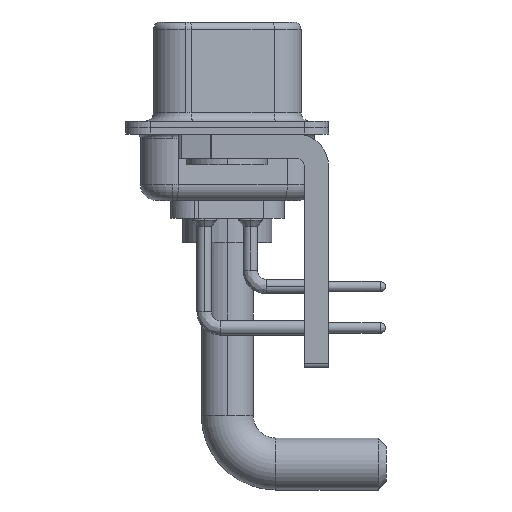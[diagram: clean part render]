
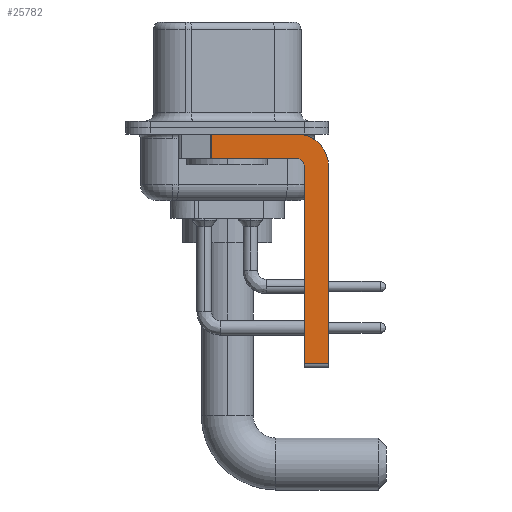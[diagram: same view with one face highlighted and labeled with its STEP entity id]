
A CAD part, left-side view. The second image highlights one B-rep face of the part: STEP entity #25782.
In plain terms, the highlighted planar face has unit normal (-1, 0, 0).
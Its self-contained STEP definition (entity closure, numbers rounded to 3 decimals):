
#176 = DIRECTION ( 'NONE',  ( -1., 0., 0. ) ) ;
#383 = EDGE_CURVE ( 'NONE', #3870, #25804, #3470, .T. ) ;
#415 = CARTESIAN_POINT ( 'NONE',  ( -2.9, -4.75, -2.4 ) ) ;
#461 = DIRECTION ( 'NONE',  ( 0., 0., 1. ) ) ;
#722 = ORIENTED_EDGE ( 'NONE', *, *, #26413, .F. ) ;
#1098 = AXIS2_PLACEMENT_3D ( 'NONE', #14844, #8532, #25747 ) ;
#1324 = CARTESIAN_POINT ( 'NONE',  ( -2.9, -4.75, -14.55 ) ) ;
#1510 = DIRECTION ( 'NONE',  ( 0., 1., 0. ) ) ;
#1531 = VERTEX_POINT ( 'NONE', #12823 ) ;
#1748 = DIRECTION ( 'NONE',  ( 1., 0., 0. ) ) ;
#1818 = EDGE_CURVE ( 'NONE', #3870, #1531, #24240, .T. ) ;
#2476 = CARTESIAN_POINT ( 'NONE',  ( -2.9, -4.25, -2.4 ) ) ;
#2653 = VERTEX_POINT ( 'NONE', #13644 ) ;
#3034 = EDGE_CURVE ( 'NONE', #9534, #18724, #16740, .T. ) ;
#3470 = LINE ( 'NONE', #15856, #16679 ) ;
#3651 = DIRECTION ( 'NONE',  ( 0., 0., -1. ) ) ;
#3870 = VERTEX_POINT ( 'NONE', #12216 ) ;
#4128 = AXIS2_PLACEMENT_3D ( 'NONE', #2476, #176, #461 ) ;
#4486 = EDGE_CURVE ( 'NONE', #1531, #2653, #14009, .T. ) ;
#4952 = AXIS2_PLACEMENT_3D ( 'NONE', #7802, #1748, #22076 ) ;
#5189 = LINE ( 'NONE', #13006, #18587 ) ;
#7802 = CARTESIAN_POINT ( 'NONE',  ( -2.9, -4.25, -2.4 ) ) ;
#7938 = VECTOR ( 'NONE', #10919, 1000. ) ;
#8532 = DIRECTION ( 'NONE',  ( 1., 0., 0. ) ) ;
#9137 = ORIENTED_EDGE ( 'NONE', *, *, #3034, .F. ) ;
#9534 = VERTEX_POINT ( 'NONE', #1324 ) ;
#10223 = ORIENTED_EDGE ( 'NONE', *, *, #23318, .F. ) ;
#10919 = DIRECTION ( 'NONE',  ( 0., 0., 1. ) ) ;
#11368 = DIRECTION ( 'NONE',  ( 0., -1., 0. ) ) ;
#11846 = EDGE_CURVE ( 'NONE', #9534, #12852, #5189, .T. ) ;
#12123 = PLANE ( 'NONE',  #4952 ) ;
#12216 = CARTESIAN_POINT ( 'NONE',  ( -2.9, 0.978, -0.4 ) ) ;
#12655 = ORIENTED_EDGE ( 'NONE', *, *, #383, .T. ) ;
#12823 = CARTESIAN_POINT ( 'NONE',  ( -2.9, -4.25, -0.4 ) ) ;
#12852 = VERTEX_POINT ( 'NONE', #14757 ) ;
#13006 = CARTESIAN_POINT ( 'NONE',  ( -2.9, -4.25, -14.55 ) ) ;
#13644 = CARTESIAN_POINT ( 'NONE',  ( -2.9, -6.25, -2.4 ) ) ;
#14009 = CIRCLE ( 'NONE', #1098, 2. ) ;
#14757 = CARTESIAN_POINT ( 'NONE',  ( -2.9, -6.25, -14.55 ) ) ;
#14844 = CARTESIAN_POINT ( 'NONE',  ( -2.9, -4.25, -2.4 ) ) ;
#15205 = EDGE_CURVE ( 'NONE', #2653, #12852, #24018, .T. ) ;
#15856 = CARTESIAN_POINT ( 'NONE',  ( -2.9, 0.978, -1.9 ) ) ;
#15955 = ORIENTED_EDGE ( 'NONE', *, *, #11846, .T. ) ;
#16017 = CARTESIAN_POINT ( 'NONE',  ( -2.9, 3., -0.4 ) ) ;
#16601 = CIRCLE ( 'NONE', #4128, 0.5 ) ;
#16617 = VERTEX_POINT ( 'NONE', #17714 ) ;
#16679 = VECTOR ( 'NONE', #23939, 1000. ) ;
#16740 = LINE ( 'NONE', #22918, #7938 ) ;
#16844 = ORIENTED_EDGE ( 'NONE', *, *, #15205, .F. ) ;
#17714 = CARTESIAN_POINT ( 'NONE',  ( -2.9, -4.25, -1.9 ) ) ;
#17895 = VECTOR ( 'NONE', #22566, 1000. ) ;
#17907 = VECTOR ( 'NONE', #1510, 1000. ) ;
#18048 = CARTESIAN_POINT ( 'NONE',  ( -2.9, 0.978, -1.9 ) ) ;
#18234 = ORIENTED_EDGE ( 'NONE', *, *, #1818, .F. ) ;
#18587 = VECTOR ( 'NONE', #11368, 1000. ) ;
#18724 = VERTEX_POINT ( 'NONE', #415 ) ;
#19371 = VECTOR ( 'NONE', #3651, 1000. ) ;
#21732 = LINE ( 'NONE', #26056, #17907 ) ;
#22076 = DIRECTION ( 'NONE',  ( 0., 0., -1. ) ) ;
#22244 = CARTESIAN_POINT ( 'NONE',  ( -2.9, -6.25, -2.4 ) ) ;
#22566 = DIRECTION ( 'NONE',  ( 0., -1., 0. ) ) ;
#22918 = CARTESIAN_POINT ( 'NONE',  ( -2.9, -4.75, -14.8 ) ) ;
#23318 = EDGE_CURVE ( 'NONE', #16617, #25804, #21732, .T. ) ;
#23830 = FACE_OUTER_BOUND ( 'NONE', #24702, .T. ) ;
#23939 = DIRECTION ( 'NONE',  ( 0., 0., -1. ) ) ;
#24018 = LINE ( 'NONE', #22244, #19371 ) ;
#24240 = LINE ( 'NONE', #16017, #17895 ) ;
#24702 = EDGE_LOOP ( 'NONE', ( #18234, #12655, #10223, #722, #9137, #15955, #16844, #26433 ) ) ;
#25747 = DIRECTION ( 'NONE',  ( 0., 0., -1. ) ) ;
#25782 = ADVANCED_FACE ( 'NONE', ( #23830 ), #12123, .F. ) ;
#25804 = VERTEX_POINT ( 'NONE', #18048 ) ;
#26056 = CARTESIAN_POINT ( 'NONE',  ( -2.9, -4.25, -1.9 ) ) ;
#26413 = EDGE_CURVE ( 'NONE', #18724, #16617, #16601, .T. ) ;
#26433 = ORIENTED_EDGE ( 'NONE', *, *, #4486, .F. ) ;
